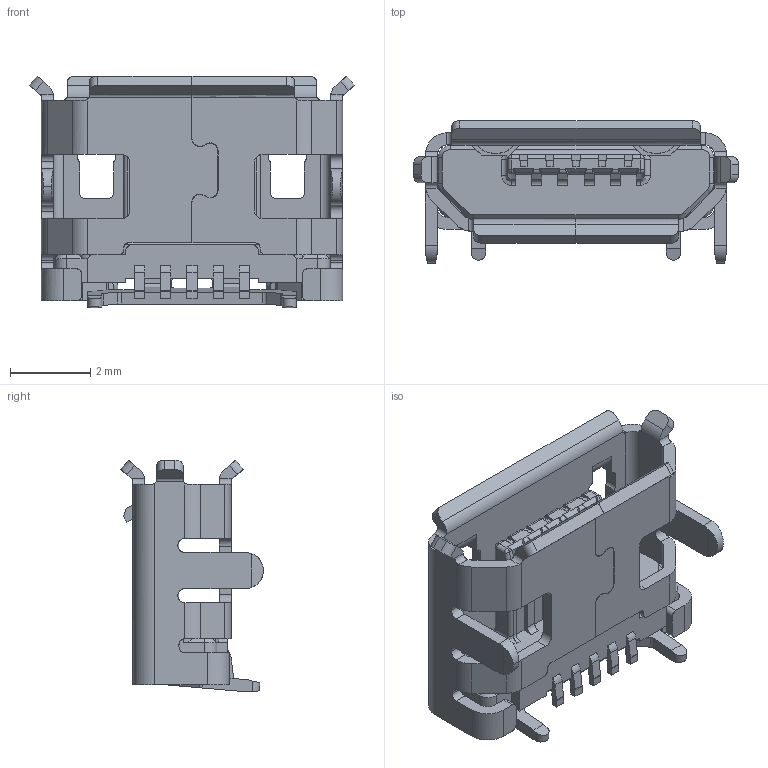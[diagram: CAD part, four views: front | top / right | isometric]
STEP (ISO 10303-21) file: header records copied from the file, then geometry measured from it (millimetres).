
FILE_DESCRIPTION (( 'STEP AP214' ), '1' );
FILE_NAME ('690T505-162-010.STEP', '2021-01-14T22:20:19', ( '' ), ( '' ), 'SwSTEP 2.0', 'SolidWorks 2020', '' );
FILE_SCHEMA (( 'AUTOMOTIVE_DESIGN' ));
Length unit declared in the file: millimetre
Products named in the file (3): SHELL 690T505-X62-01X; Insulator 690T505-X62-01X_WHITE; 690T505-162-010
Assembly tree (2 placements, depth 2):
  690T505-162-010
    Insulator 690T505-X62-01X_WHITE
    SHELL 690T505-X62-01X
Bounding box: 8.1 x 3.55 x 5.77 mm (x, y, z)
Volume: 43.2 mm3; surface area: 278.5 mm2
Topology: 2 solids, 2 shells, 653 faces, 1839 edges, 1190 vertices
Faces by surface type: plane 415, cylinder 199, bspline 23, cone 16
Entity records: 22964 total; most frequent: CARTESIAN_POINT 6577, ORIENTED_EDGE 3670, DIRECTION 2708, EDGE_CURVE 1835, VERTEX_POINT 1190, LINE 1168, VECTOR 1168, AXIS2_PLACEMENT_3D 770
